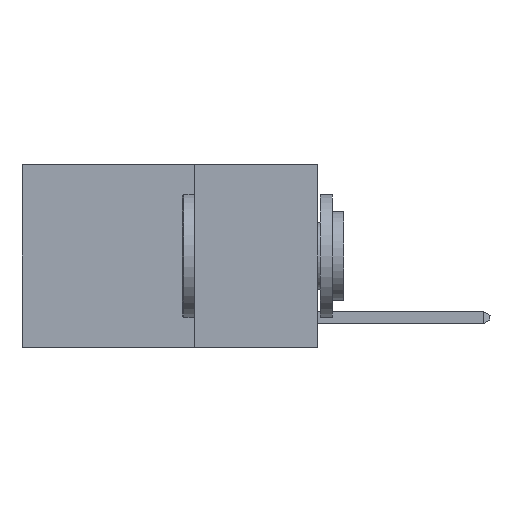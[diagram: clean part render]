
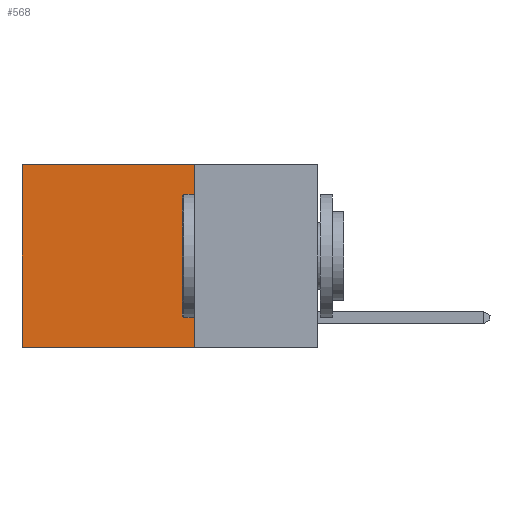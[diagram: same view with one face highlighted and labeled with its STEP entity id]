
A CAD part, left-side view. The second image highlights one B-rep face of the part: STEP entity #568.
In plain terms, the highlighted planar face has unit normal (-1, 0, 0).
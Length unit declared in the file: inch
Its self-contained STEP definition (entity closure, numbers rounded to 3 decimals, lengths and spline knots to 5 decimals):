
#33 = CARTESIAN_POINT ( 'NONE',  ( 0.2625, 0.25, 0. ) ) ;
#291 = CARTESIAN_POINT ( 'NONE',  ( 0.2625, 0.25, 0. ) ) ;
#566 = VERTEX_POINT ( 'NONE', #9415 ) ;
#568 = ADVANCED_FACE ( 'NONE', ( #1773 ), #7675, .F. ) ;
#902 = ORIENTED_EDGE ( 'NONE', *, *, #3151, .F. ) ;
#1340 = CARTESIAN_POINT ( 'NONE',  ( 0.2625, 0.25, 0. ) ) ;
#1427 = EDGE_CURVE ( 'NONE', #6480, #566, #3669, .T. ) ;
#1648 = ORIENTED_EDGE ( 'NONE', *, *, #8436, .T. ) ;
#1773 = FACE_OUTER_BOUND ( 'NONE', #3505, .T. ) ;
#2552 = VECTOR ( 'NONE', #12091, 39.37008 ) ;
#3151 = EDGE_CURVE ( 'NONE', #3614, #8862, #6767, .T. ) ;
#3298 = CARTESIAN_POINT ( 'NONE',  ( 0.2625, 0.6, 0. ) ) ;
#3505 = EDGE_LOOP ( 'NONE', ( #10430, #8594, #902, #1648 ) ) ;
#3614 = VERTEX_POINT ( 'NONE', #291 ) ;
#3669 = LINE ( 'NONE', #8362, #2552 ) ;
#5977 = EDGE_CURVE ( 'NONE', #8862, #566, #12471, .T. ) ;
#6050 = AXIS2_PLACEMENT_3D ( 'NONE', #33, #8942, #11679 ) ;
#6480 = VERTEX_POINT ( 'NONE', #3298 ) ;
#6544 = VECTOR ( 'NONE', #8761, 39.37008 ) ;
#6767 = LINE ( 'NONE', #9642, #6544 ) ;
#7242 = DIRECTION ( 'NONE',  ( 0., 1., 0. ) ) ;
#7675 = PLANE ( 'NONE',  #6050 ) ;
#7787 = VECTOR ( 'NONE', #7242, 39.37008 ) ;
#8362 = CARTESIAN_POINT ( 'NONE',  ( 0.2625, 0.6, 0. ) ) ;
#8436 = EDGE_CURVE ( 'NONE', #3614, #6480, #10233, .T. ) ;
#8594 = ORIENTED_EDGE ( 'NONE', *, *, #5977, .F. ) ;
#8761 = DIRECTION ( 'NONE',  ( 0., 0., -1. ) ) ;
#8862 = VERTEX_POINT ( 'NONE', #10778 ) ;
#8942 = DIRECTION ( 'NONE',  ( 1., 0., 0. ) ) ;
#9415 = CARTESIAN_POINT ( 'NONE',  ( 0.2625, 0.6, -0.37 ) ) ;
#9642 = CARTESIAN_POINT ( 'NONE',  ( 0.2625, 0.25, 0. ) ) ;
#9726 = DIRECTION ( 'NONE',  ( 0., 1., 0. ) ) ;
#10233 = LINE ( 'NONE', #1340, #7787 ) ;
#10430 = ORIENTED_EDGE ( 'NONE', *, *, #1427, .T. ) ;
#10778 = CARTESIAN_POINT ( 'NONE',  ( 0.2625, 0.25, -0.37 ) ) ;
#11679 = DIRECTION ( 'NONE',  ( 0., 0., -1. ) ) ;
#12007 = VECTOR ( 'NONE', #9726, 39.37008 ) ;
#12091 = DIRECTION ( 'NONE',  ( 0., 0., -1. ) ) ;
#12471 = LINE ( 'NONE', #12539, #12007 ) ;
#12539 = CARTESIAN_POINT ( 'NONE',  ( 0.2625, 0.25, -0.37 ) ) ;
